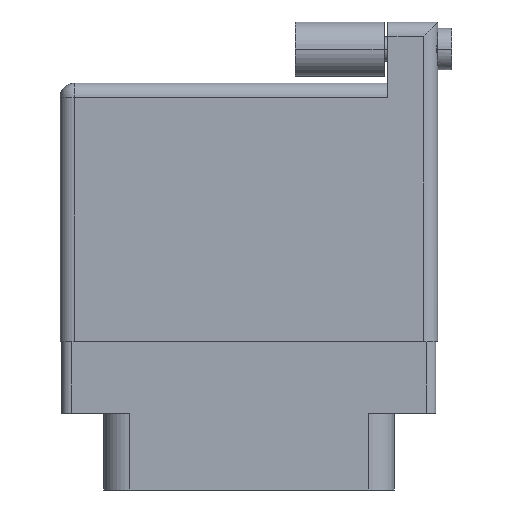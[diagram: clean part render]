
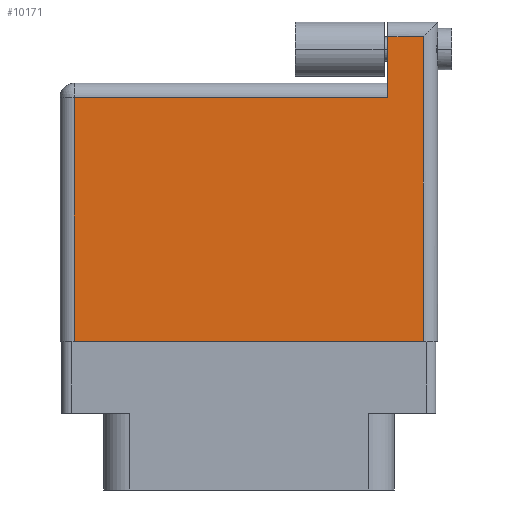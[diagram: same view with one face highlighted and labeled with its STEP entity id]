
A CAD part, front view. The second image highlights one B-rep face of the part: STEP entity #10171.
In plain terms, the highlighted face is planar.
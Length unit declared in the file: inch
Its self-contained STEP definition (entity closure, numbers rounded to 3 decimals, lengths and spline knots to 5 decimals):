
#155 = VECTOR ( 'NONE', #4347, 39.37008 ) ;
#320 = ORIENTED_EDGE ( 'NONE', *, *, #1346, .T. ) ;
#736 = VECTOR ( 'NONE', #7306, 39.37008 ) ;
#1205 = AXIS2_PLACEMENT_3D ( 'NONE', #2585, #11958, #15353 ) ;
#1346 = EDGE_CURVE ( 'NONE', #6847, #2447, #9152, .T. ) ;
#1651 = EDGE_LOOP ( 'NONE', ( #3490, #21586, #20911, #9550, #16753, #320 ) ) ;
#2447 = VERTEX_POINT ( 'NONE', #7350 ) ;
#2585 = CARTESIAN_POINT ( 'NONE',  ( 0., 0.906, 0. ) ) ;
#3370 = LINE ( 'NONE', #14040, #736 ) ;
#3490 = ORIENTED_EDGE ( 'NONE', *, *, #16109, .T. ) ;
#3533 = LINE ( 'NONE', #8440, #19713 ) ;
#4347 = DIRECTION ( 'NONE',  ( 0., -1., 0. ) ) ;
#5040 = EDGE_CURVE ( 'NONE', #6569, #6740, #8404, .T. ) ;
#5127 = CARTESIAN_POINT ( 'NONE',  ( 1.15, 1.12, 0. ) ) ;
#6030 = VECTOR ( 'NONE', #10244, 39.37008 ) ;
#6569 = VERTEX_POINT ( 'NONE', #19780 ) ;
#6740 = VERTEX_POINT ( 'NONE', #17412 ) ;
#6847 = VERTEX_POINT ( 'NONE', #17262 ) ;
#7306 = DIRECTION ( 'NONE',  ( -1., 0., 0. ) ) ;
#7350 = CARTESIAN_POINT ( 'NONE',  ( 0.05, 0., 0. ) ) ;
#7470 = EDGE_CURVE ( 'NONE', #13701, #6569, #3533, .T. ) ;
#8404 = LINE ( 'NONE', #5127, #6030 ) ;
#8440 = CARTESIAN_POINT ( 'NONE',  ( 0., 1.07, 0. ) ) ;
#9152 = LINE ( 'NONE', #14503, #155 ) ;
#9550 = ORIENTED_EDGE ( 'NONE', *, *, #5040, .T. ) ;
#10171 = ADVANCED_FACE ( 'NONE', ( #21991 ), #15166, .F. ) ;
#10244 = DIRECTION ( 'NONE',  ( 0., -1., 0. ) ) ;
#10552 = VECTOR ( 'NONE', #12514, 39.37008 ) ;
#10607 = CARTESIAN_POINT ( 'NONE',  ( 1.275, 1.12, 0. ) ) ;
#10897 = DIRECTION ( 'NONE',  ( 0., 1., 0. ) ) ;
#11006 = EDGE_CURVE ( 'NONE', #6740, #6847, #3370, .T. ) ;
#11133 = CARTESIAN_POINT ( 'NONE',  ( 1.275, 1.07, 0. ) ) ;
#11958 = DIRECTION ( 'NONE',  ( 0., 0., -1. ) ) ;
#12179 = EDGE_CURVE ( 'NONE', #19449, #13701, #19239, .T. ) ;
#12514 = DIRECTION ( 'NONE',  ( 1., 0., 0. ) ) ;
#12590 = VECTOR ( 'NONE', #10897, 39.37008 ) ;
#13701 = VERTEX_POINT ( 'NONE', #11133 ) ;
#14040 = CARTESIAN_POINT ( 'NONE',  ( 0., 0.856, 0. ) ) ;
#14454 = CARTESIAN_POINT ( 'NONE',  ( 1.275, 0., 0. ) ) ;
#14503 = CARTESIAN_POINT ( 'NONE',  ( 0.05, 0., 0. ) ) ;
#14513 = CARTESIAN_POINT ( 'NONE',  ( 0., 0., 0. ) ) ;
#15166 = PLANE ( 'NONE',  #1205 ) ;
#15353 = DIRECTION ( 'NONE',  ( -1., 0., 0. ) ) ;
#16109 = EDGE_CURVE ( 'NONE', #2447, #19449, #17737, .T. ) ;
#16753 = ORIENTED_EDGE ( 'NONE', *, *, #11006, .T. ) ;
#17262 = CARTESIAN_POINT ( 'NONE',  ( 0.05, 0.856, 0. ) ) ;
#17412 = CARTESIAN_POINT ( 'NONE',  ( 1.15, 0.856, 0. ) ) ;
#17737 = LINE ( 'NONE', #14513, #10552 ) ;
#19239 = LINE ( 'NONE', #10607, #12590 ) ;
#19449 = VERTEX_POINT ( 'NONE', #14454 ) ;
#19713 = VECTOR ( 'NONE', #20319, 39.37008 ) ;
#19780 = CARTESIAN_POINT ( 'NONE',  ( 1.15, 1.07, 0. ) ) ;
#20319 = DIRECTION ( 'NONE',  ( -1., 0., 0. ) ) ;
#20911 = ORIENTED_EDGE ( 'NONE', *, *, #7470, .T. ) ;
#21586 = ORIENTED_EDGE ( 'NONE', *, *, #12179, .T. ) ;
#21991 = FACE_OUTER_BOUND ( 'NONE', #1651, .T. ) ;
